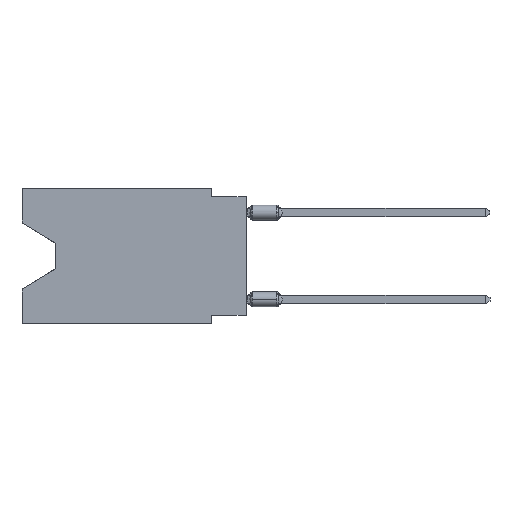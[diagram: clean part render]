
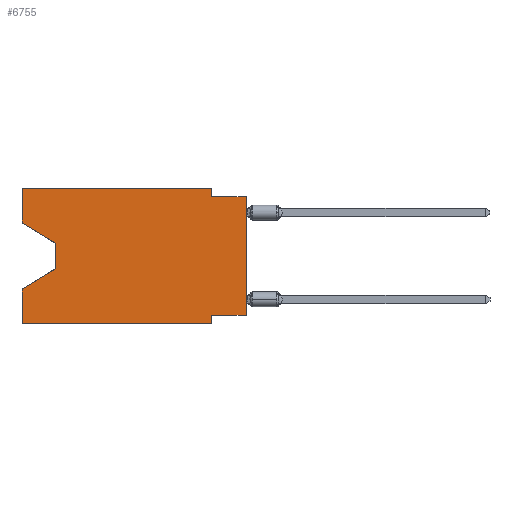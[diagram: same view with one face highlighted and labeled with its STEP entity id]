
A CAD part, left-side view. The second image highlights one B-rep face of the part: STEP entity #6755.
In plain terms, the highlighted planar face has unit normal (-1, 0, 0).
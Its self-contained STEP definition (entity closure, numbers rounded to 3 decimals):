
#59 = VERTEX_POINT ( 'NONE', #9864 ) ;
#203 = EDGE_CURVE ( 'NONE', #4402, #2071, #12152, .T. ) ;
#377 = VERTEX_POINT ( 'NONE', #8487 ) ;
#631 = DIRECTION ( 'NONE',  ( 0., -1., 0. ) ) ;
#701 = VECTOR ( 'NONE', #12090, 1000. ) ;
#715 = CARTESIAN_POINT ( 'NONE',  ( 0., 0., -0.635 ) ) ;
#734 = LINE ( 'NONE', #7589, #8164 ) ;
#817 = EDGE_LOOP ( 'NONE', ( #2609, #2739, #1927, #8841, #2591, #11362, #6350, #11303, #3007, #9942, #6366, #11464 ) ) ;
#824 = EDGE_CURVE ( 'NONE', #11032, #6616, #3407, .T. ) ;
#1109 = PLANE ( 'NONE',  #8547 ) ;
#1222 = EDGE_CURVE ( 'NONE', #377, #11032, #734, .T. ) ;
#1311 = DIRECTION ( 'NONE',  ( 1., 0., 0. ) ) ;
#1365 = CARTESIAN_POINT ( 'NONE',  ( 0., 16.383, 0. ) ) ;
#1390 = EDGE_CURVE ( 'NONE', #3324, #8011, #7874, .T. ) ;
#1643 = DIRECTION ( 'NONE',  ( 0., 0., 1. ) ) ;
#1866 = EDGE_CURVE ( 'NONE', #377, #3324, #11304, .T. ) ;
#1870 = VECTOR ( 'NONE', #11369, 1000. ) ;
#1874 = LINE ( 'NONE', #9954, #11418 ) ;
#1927 = ORIENTED_EDGE ( 'NONE', *, *, #4942, .T. ) ;
#2012 = CARTESIAN_POINT ( 'NONE',  ( 0., 16.383, 0. ) ) ;
#2071 = VERTEX_POINT ( 'NONE', #3809 ) ;
#2122 = VECTOR ( 'NONE', #5947, 1000. ) ;
#2544 = CARTESIAN_POINT ( 'NONE',  ( 0., 13.97, -4.013 ) ) ;
#2591 = ORIENTED_EDGE ( 'NONE', *, *, #5566, .T. ) ;
#2609 = ORIENTED_EDGE ( 'NONE', *, *, #1866, .T. ) ;
#2739 = ORIENTED_EDGE ( 'NONE', *, *, #1390, .T. ) ;
#2863 = CARTESIAN_POINT ( 'NONE',  ( 0., 0., -0.635 ) ) ;
#3007 = ORIENTED_EDGE ( 'NONE', *, *, #11533, .F. ) ;
#3288 = CARTESIAN_POINT ( 'NONE',  ( 0., 16.383, -2.546 ) ) ;
#3293 = CARTESIAN_POINT ( 'NONE',  ( 0., 0., -9.271 ) ) ;
#3324 = VERTEX_POINT ( 'NONE', #11506 ) ;
#3407 = LINE ( 'NONE', #8602, #6255 ) ;
#3700 = VECTOR ( 'NONE', #6313, 1000. ) ;
#3809 = CARTESIAN_POINT ( 'NONE',  ( 0., 2.54, -9.271 ) ) ;
#4402 = VERTEX_POINT ( 'NONE', #11247 ) ;
#4609 = CARTESIAN_POINT ( 'NONE',  ( 0., 0., 0. ) ) ;
#4740 = VECTOR ( 'NONE', #10549, 1000. ) ;
#4761 = VERTEX_POINT ( 'NONE', #10314 ) ;
#4942 = EDGE_CURVE ( 'NONE', #8011, #6935, #7503, .T. ) ;
#5327 = FACE_OUTER_BOUND ( 'NONE', #817, .T. ) ;
#5566 = EDGE_CURVE ( 'NONE', #11149, #4761, #9331, .T. ) ;
#5769 = VERTEX_POINT ( 'NONE', #715 ) ;
#5947 = DIRECTION ( 'NONE',  ( 0., 0., -1. ) ) ;
#6014 = LINE ( 'NONE', #2863, #12180 ) ;
#6255 = VECTOR ( 'NONE', #631, 1000. ) ;
#6313 = DIRECTION ( 'NONE',  ( 0., -0.855, -0.519 ) ) ;
#6350 = ORIENTED_EDGE ( 'NONE', *, *, #203, .F. ) ;
#6366 = ORIENTED_EDGE ( 'NONE', *, *, #824, .F. ) ;
#6616 = VERTEX_POINT ( 'NONE', #9930 ) ;
#6755 = ADVANCED_FACE ( 'NONE', ( #5327 ), #1109, .F. ) ;
#6790 = LINE ( 'NONE', #4609, #8065 ) ;
#6935 = VERTEX_POINT ( 'NONE', #8552 ) ;
#7089 = VECTOR ( 'NONE', #9384, 1000. ) ;
#7204 = VECTOR ( 'NONE', #9783, 1000. ) ;
#7374 = CARTESIAN_POINT ( 'NONE',  ( 0., 16.383, 0. ) ) ;
#7441 = EDGE_CURVE ( 'NONE', #11149, #6935, #7625, .T. ) ;
#7503 = LINE ( 'NONE', #12540, #7204 ) ;
#7589 = CARTESIAN_POINT ( 'NONE',  ( 0., 16.383, 0. ) ) ;
#7625 = LINE ( 'NONE', #1365, #7089 ) ;
#7803 = CARTESIAN_POINT ( 'NONE',  ( 0., 2.54, -9.906 ) ) ;
#7874 = LINE ( 'NONE', #2544, #4740 ) ;
#8011 = VERTEX_POINT ( 'NONE', #9334 ) ;
#8065 = VECTOR ( 'NONE', #1643, 1000. ) ;
#8164 = VECTOR ( 'NONE', #9675, 1000. ) ;
#8487 = CARTESIAN_POINT ( 'NONE',  ( 0., 16.383, -2.546 ) ) ;
#8547 = AXIS2_PLACEMENT_3D ( 'NONE', #7374, #1311, #12215 ) ;
#8552 = CARTESIAN_POINT ( 'NONE',  ( 0., 16.383, -7.36 ) ) ;
#8602 = CARTESIAN_POINT ( 'NONE',  ( 0., 16.383, 0. ) ) ;
#8841 = ORIENTED_EDGE ( 'NONE', *, *, #7441, .F. ) ;
#8974 = DIRECTION ( 'NONE',  ( 0., 0., -1. ) ) ;
#9266 = CARTESIAN_POINT ( 'NONE',  ( 0., 16.383, -9.906 ) ) ;
#9331 = LINE ( 'NONE', #9266, #701 ) ;
#9334 = CARTESIAN_POINT ( 'NONE',  ( 0., 13.97, -5.893 ) ) ;
#9384 = DIRECTION ( 'NONE',  ( 0., 0., 1. ) ) ;
#9399 = EDGE_CURVE ( 'NONE', #4402, #5769, #6790, .T. ) ;
#9675 = DIRECTION ( 'NONE',  ( 0., 0., 1. ) ) ;
#9783 = DIRECTION ( 'NONE',  ( 0., 0.855, -0.519 ) ) ;
#9822 = LINE ( 'NONE', #7803, #2122 ) ;
#9864 = CARTESIAN_POINT ( 'NONE',  ( 0., 2.54, -0.635 ) ) ;
#9930 = CARTESIAN_POINT ( 'NONE',  ( 0., 2.54, 0. ) ) ;
#9942 = ORIENTED_EDGE ( 'NONE', *, *, #12706, .F. ) ;
#9954 = CARTESIAN_POINT ( 'NONE',  ( 0., 2.54, 0. ) ) ;
#10314 = CARTESIAN_POINT ( 'NONE',  ( 0., 2.54, -9.906 ) ) ;
#10372 = EDGE_CURVE ( 'NONE', #2071, #4761, #9822, .T. ) ;
#10549 = DIRECTION ( 'NONE',  ( 0., 0., -1. ) ) ;
#10883 = DIRECTION ( 'NONE',  ( 0., -1., 0. ) ) ;
#11032 = VERTEX_POINT ( 'NONE', #2012 ) ;
#11149 = VERTEX_POINT ( 'NONE', #12918 ) ;
#11247 = CARTESIAN_POINT ( 'NONE',  ( 0., 0., -9.271 ) ) ;
#11303 = ORIENTED_EDGE ( 'NONE', *, *, #9399, .T. ) ;
#11304 = LINE ( 'NONE', #3288, #3700 ) ;
#11362 = ORIENTED_EDGE ( 'NONE', *, *, #10372, .F. ) ;
#11369 = DIRECTION ( 'NONE',  ( 0., 1., 0. ) ) ;
#11418 = VECTOR ( 'NONE', #8974, 1000. ) ;
#11464 = ORIENTED_EDGE ( 'NONE', *, *, #1222, .F. ) ;
#11506 = CARTESIAN_POINT ( 'NONE',  ( 0., 13.97, -4.013 ) ) ;
#11533 = EDGE_CURVE ( 'NONE', #59, #5769, #6014, .T. ) ;
#12090 = DIRECTION ( 'NONE',  ( 0., -1., 0. ) ) ;
#12152 = LINE ( 'NONE', #3293, #1870 ) ;
#12180 = VECTOR ( 'NONE', #10883, 1000. ) ;
#12215 = DIRECTION ( 'NONE',  ( 0., 0., -1. ) ) ;
#12540 = CARTESIAN_POINT ( 'NONE',  ( 0., 13.97, -5.893 ) ) ;
#12706 = EDGE_CURVE ( 'NONE', #6616, #59, #1874, .T. ) ;
#12918 = CARTESIAN_POINT ( 'NONE',  ( 0., 16.383, -9.906 ) ) ;
